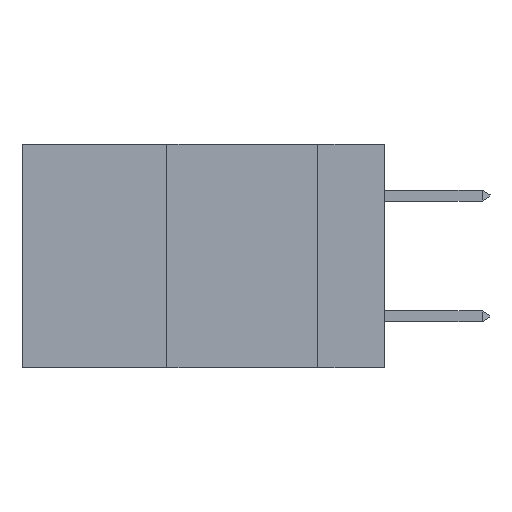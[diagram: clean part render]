
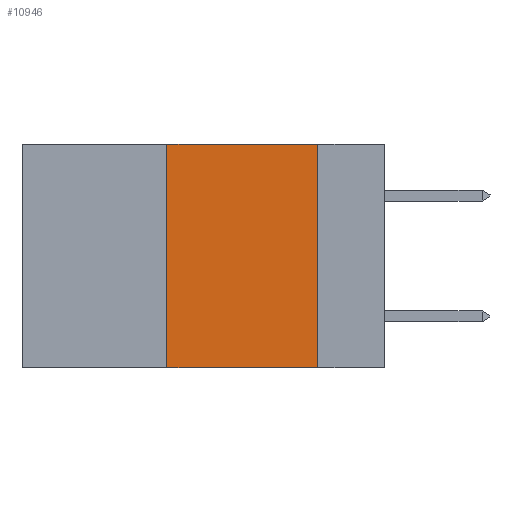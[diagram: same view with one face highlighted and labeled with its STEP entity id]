
A CAD part, left-side view. The second image highlights one B-rep face of the part: STEP entity #10946.
In plain terms, the highlighted planar face has unit normal (-1, 0, 0).
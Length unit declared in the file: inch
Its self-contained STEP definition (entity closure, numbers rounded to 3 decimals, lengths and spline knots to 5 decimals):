
#387 = VERTEX_POINT ( 'NONE', #11347 ) ;
#939 = CARTESIAN_POINT ( 'NONE',  ( 0., 0.36, 0. ) ) ;
#996 = EDGE_LOOP ( 'NONE', ( #9249, #5826, #9342, #3554 ) ) ;
#1379 = DIRECTION ( 'NONE',  ( 0., 0., 1. ) ) ;
#2039 = EDGE_CURVE ( 'NONE', #2633, #6283, #5053, .T. ) ;
#2633 = VERTEX_POINT ( 'NONE', #939 ) ;
#2923 = FACE_OUTER_BOUND ( 'NONE', #996, .T. ) ;
#3002 = AXIS2_PLACEMENT_3D ( 'NONE', #8816, #4255, #10525 ) ;
#3340 = PLANE ( 'NONE',  #3002 ) ;
#3554 = ORIENTED_EDGE ( 'NONE', *, *, #10642, .T. ) ;
#3626 = CARTESIAN_POINT ( 'NONE',  ( 0., 0.6, -0.37 ) ) ;
#4255 = DIRECTION ( 'NONE',  ( 1., 0., 0. ) ) ;
#4792 = VECTOR ( 'NONE', #9923, 39.37008 ) ;
#4967 = CARTESIAN_POINT ( 'NONE',  ( 0., 0.11, 0. ) ) ;
#5053 = LINE ( 'NONE', #5427, #7244 ) ;
#5427 = CARTESIAN_POINT ( 'NONE',  ( 0., 0.6, 0. ) ) ;
#5723 = CARTESIAN_POINT ( 'NONE',  ( 0., 0.11, -0.37 ) ) ;
#5826 = ORIENTED_EDGE ( 'NONE', *, *, #2039, .F. ) ;
#6283 = VERTEX_POINT ( 'NONE', #11507 ) ;
#6931 = VERTEX_POINT ( 'NONE', #5723 ) ;
#7123 = VECTOR ( 'NONE', #1379, 39.37008 ) ;
#7179 = VECTOR ( 'NONE', #11216, 39.37008 ) ;
#7244 = VECTOR ( 'NONE', #9486, 39.37008 ) ;
#8330 = EDGE_CURVE ( 'NONE', #6283, #6931, #8725, .T. ) ;
#8725 = LINE ( 'NONE', #4967, #7179 ) ;
#8751 = CARTESIAN_POINT ( 'NONE',  ( 0., 0.36, 0. ) ) ;
#8816 = CARTESIAN_POINT ( 'NONE',  ( 0., 0.6, 0. ) ) ;
#9249 = ORIENTED_EDGE ( 'NONE', *, *, #8330, .F. ) ;
#9342 = ORIENTED_EDGE ( 'NONE', *, *, #10385, .F. ) ;
#9471 = LINE ( 'NONE', #8751, #7123 ) ;
#9486 = DIRECTION ( 'NONE',  ( 0., -1., 0. ) ) ;
#9923 = DIRECTION ( 'NONE',  ( 0., -1., 0. ) ) ;
#10385 = EDGE_CURVE ( 'NONE', #387, #2633, #9471, .T. ) ;
#10525 = DIRECTION ( 'NONE',  ( 0., 0., -1. ) ) ;
#10642 = EDGE_CURVE ( 'NONE', #387, #6931, #11366, .T. ) ;
#10946 = ADVANCED_FACE ( 'NONE', ( #2923 ), #3340, .F. ) ;
#11216 = DIRECTION ( 'NONE',  ( 0., 0., -1. ) ) ;
#11347 = CARTESIAN_POINT ( 'NONE',  ( 0., 0.36, -0.37 ) ) ;
#11366 = LINE ( 'NONE', #3626, #4792 ) ;
#11507 = CARTESIAN_POINT ( 'NONE',  ( 0., 0.11, 0. ) ) ;
